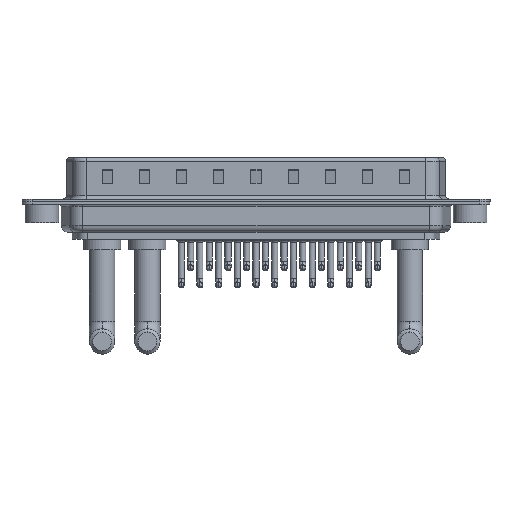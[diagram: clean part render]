
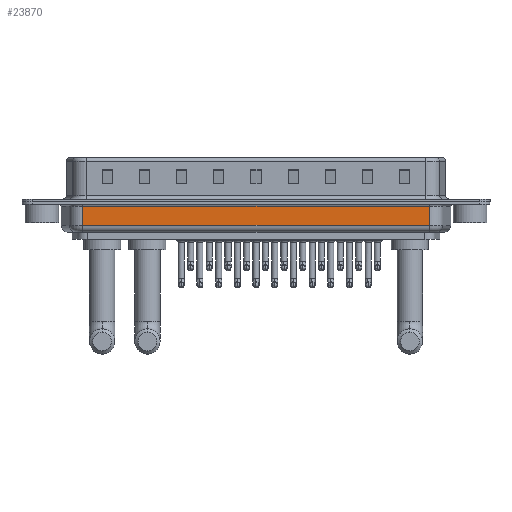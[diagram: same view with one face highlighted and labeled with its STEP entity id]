
A CAD part, front view. The second image highlights one B-rep face of the part: STEP entity #23870.
In plain terms, the highlighted planar face has unit normal (0, -1, 0).
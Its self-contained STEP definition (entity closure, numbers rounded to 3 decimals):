
#1244 = VECTOR ( 'NONE', #21130, 1000. ) ;
#1509 = EDGE_CURVE ( 'NONE', #27561, #7980, #17879, .T. ) ;
#2174 = ORIENTED_EDGE ( 'NONE', *, *, #1509, .T. ) ;
#2672 = VECTOR ( 'NONE', #18855, 1000. ) ;
#4138 = DIRECTION ( 'NONE',  ( 0., 1., 0. ) ) ;
#4612 = LINE ( 'NONE', #6328, #20432 ) ;
#4781 = EDGE_CURVE ( 'NONE', #7980, #5943, #4612, .T. ) ;
#5640 = EDGE_CURVE ( 'NONE', #8239, #5943, #23114, .T. ) ;
#5943 = VERTEX_POINT ( 'NONE', #9209 ) ;
#6328 = CARTESIAN_POINT ( 'NONE',  ( 6.031, -5.35, -0.65 ) ) ;
#6524 = CARTESIAN_POINT ( 'NONE',  ( 6.031, -5.35, -4.5 ) ) ;
#7980 = VERTEX_POINT ( 'NONE', #22813 ) ;
#8203 = ORIENTED_EDGE ( 'NONE', *, *, #5640, .F. ) ;
#8239 = VERTEX_POINT ( 'NONE', #22513 ) ;
#9209 = CARTESIAN_POINT ( 'NONE',  ( 6.031, -5.35, -0.65 ) ) ;
#10792 = FACE_OUTER_BOUND ( 'NONE', #25829, .T. ) ;
#11120 = VECTOR ( 'NONE', #24694, 1000. ) ;
#12225 = CARTESIAN_POINT ( 'NONE',  ( 6.031, -5.35, -3.5 ) ) ;
#12504 = LINE ( 'NONE', #12225, #1244 ) ;
#13498 = CARTESIAN_POINT ( 'NONE',  ( 57.469, -5.35, -3.5 ) ) ;
#16553 = ORIENTED_EDGE ( 'NONE', *, *, #20574, .T. ) ;
#17879 = LINE ( 'NONE', #20565, #11120 ) ;
#18855 = DIRECTION ( 'NONE',  ( 0., 0., 1. ) ) ;
#19011 = PLANE ( 'NONE',  #21858 ) ;
#20432 = VECTOR ( 'NONE', #23720, 1000. ) ;
#20565 = CARTESIAN_POINT ( 'NONE',  ( 57.469, -5.35, -4.5 ) ) ;
#20574 = EDGE_CURVE ( 'NONE', #8239, #27561, #12504, .T. ) ;
#20974 = CARTESIAN_POINT ( 'NONE',  ( 6.031, -5.35, -4.5 ) ) ;
#21130 = DIRECTION ( 'NONE',  ( 1., 0., 0. ) ) ;
#21858 = AXIS2_PLACEMENT_3D ( 'NONE', #6524, #4138, #26068 ) ;
#22513 = CARTESIAN_POINT ( 'NONE',  ( 6.031, -5.35, -3.5 ) ) ;
#22813 = CARTESIAN_POINT ( 'NONE',  ( 57.469, -5.35, -0.65 ) ) ;
#23114 = LINE ( 'NONE', #20974, #2672 ) ;
#23720 = DIRECTION ( 'NONE',  ( -1., 0., 0. ) ) ;
#23870 = ADVANCED_FACE ( 'NONE', ( #10792 ), #19011, .F. ) ;
#24694 = DIRECTION ( 'NONE',  ( 0., 0., 1. ) ) ;
#25829 = EDGE_LOOP ( 'NONE', ( #8203, #16553, #2174, #26537 ) ) ;
#26068 = DIRECTION ( 'NONE',  ( -1., 0., 0. ) ) ;
#26537 = ORIENTED_EDGE ( 'NONE', *, *, #4781, .T. ) ;
#27561 = VERTEX_POINT ( 'NONE', #13498 ) ;
